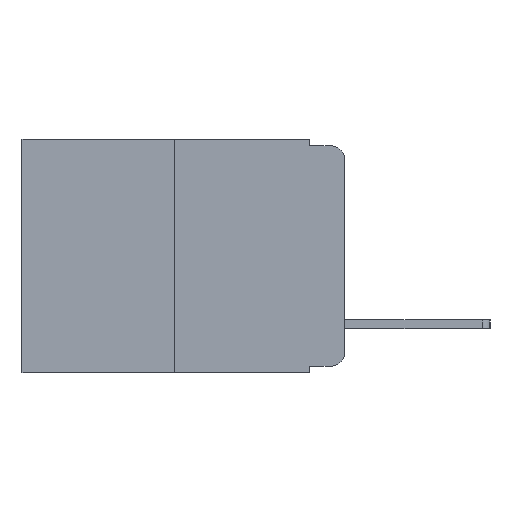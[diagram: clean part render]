
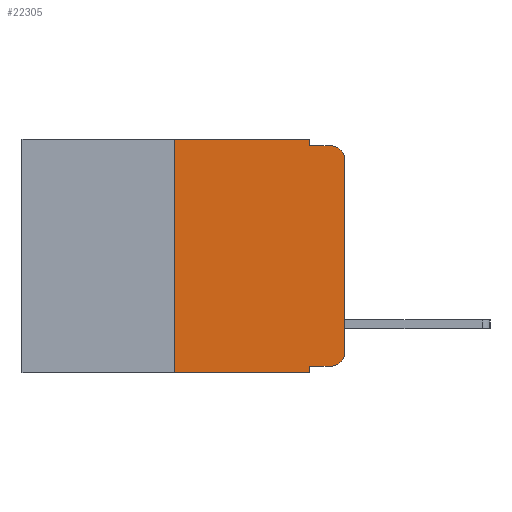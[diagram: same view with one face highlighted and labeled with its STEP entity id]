
A CAD part, left-side view. The second image highlights one B-rep face of the part: STEP entity #22305.
In plain terms, the highlighted planar face has unit normal (-1, 0, 0).
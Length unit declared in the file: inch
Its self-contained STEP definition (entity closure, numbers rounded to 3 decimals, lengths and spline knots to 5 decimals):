
#561 = DIRECTION ( 'NONE',  ( 0., 0., -1. ) ) ;
#583 = DIRECTION ( 'NONE',  ( 0., 0., -1. ) ) ;
#586 = ORIENTED_EDGE ( 'NONE', *, *, #11190, .T. ) ;
#628 = FACE_OUTER_BOUND ( 'NONE', #15506, .T. ) ;
#839 = VECTOR ( 'NONE', #18678, 39.37008 ) ;
#875 = VECTOR ( 'NONE', #18626, 39.37008 ) ;
#943 = VERTEX_POINT ( 'NONE', #12733 ) ;
#1060 = EDGE_CURVE ( 'NONE', #22845, #11990, #15391, .T. ) ;
#1147 = VERTEX_POINT ( 'NONE', #21164 ) ;
#1236 = CARTESIAN_POINT ( 'NONE',  ( 0., 0.473, 0. ) ) ;
#1577 = VECTOR ( 'NONE', #11645, 39.37008 ) ;
#2353 = VERTEX_POINT ( 'NONE', #16899 ) ;
#3320 = ORIENTED_EDGE ( 'NONE', *, *, #8495, .T. ) ;
#3538 = DIRECTION ( 'NONE',  ( 0., 0., 1. ) ) ;
#3705 = ORIENTED_EDGE ( 'NONE', *, *, #23153, .F. ) ;
#3804 = VERTEX_POINT ( 'NONE', #5965 ) ;
#3935 = CARTESIAN_POINT ( 'NONE',  ( 0., 0.25, 0. ) ) ;
#3940 = DIRECTION ( 'NONE',  ( 0., 0., -1. ) ) ;
#4146 = CARTESIAN_POINT ( 'NONE',  ( 0., 0.051, 0. ) ) ;
#4172 = ORIENTED_EDGE ( 'NONE', *, *, #20846, .T. ) ;
#4458 = CARTESIAN_POINT ( 'NONE',  ( 0., 0.051, -0.333 ) ) ;
#4503 = VERTEX_POINT ( 'NONE', #22174 ) ;
#4615 = ORIENTED_EDGE ( 'NONE', *, *, #7274, .F. ) ;
#4837 = EDGE_CURVE ( 'NONE', #2353, #1147, #15476, .T. ) ;
#5032 = ORIENTED_EDGE ( 'NONE', *, *, #19635, .T. ) ;
#5465 = CARTESIAN_POINT ( 'NONE',  ( 0., 0.25, 0. ) ) ;
#5498 = VERTEX_POINT ( 'NONE', #23075 ) ;
#5540 = LINE ( 'NONE', #11544, #10066 ) ;
#5965 = CARTESIAN_POINT ( 'NONE',  ( 0., 0.051, -0.333 ) ) ;
#6021 = CIRCLE ( 'NONE', #8492, 0.02 ) ;
#6303 = DIRECTION ( 'NONE',  ( 0., -1., 0. ) ) ;
#6677 = CARTESIAN_POINT ( 'NONE',  ( 0., 0.02, -0.313 ) ) ;
#7274 = EDGE_CURVE ( 'NONE', #1147, #11995, #19494, .T. ) ;
#7289 = CARTESIAN_POINT ( 'NONE',  ( 0., 0.02, -0.01 ) ) ;
#7557 = CARTESIAN_POINT ( 'NONE',  ( 0., 0.473, 0. ) ) ;
#7959 = VECTOR ( 'NONE', #3538, 39.37008 ) ;
#7970 = CARTESIAN_POINT ( 'NONE',  ( 0., 0.051, -0.01 ) ) ;
#8492 = AXIS2_PLACEMENT_3D ( 'NONE', #6677, #19140, #8506 ) ;
#8495 = EDGE_CURVE ( 'NONE', #943, #11995, #12582, .T. ) ;
#8506 = DIRECTION ( 'NONE',  ( 0., 0., -1. ) ) ;
#9027 = LINE ( 'NONE', #1236, #23147 ) ;
#9638 = VERTEX_POINT ( 'NONE', #10764 ) ;
#10066 = VECTOR ( 'NONE', #583, 39.37008 ) ;
#10335 = ORIENTED_EDGE ( 'NONE', *, *, #1060, .F. ) ;
#10497 = ORIENTED_EDGE ( 'NONE', *, *, #10884, .T. ) ;
#10678 = VECTOR ( 'NONE', #15025, 39.37008 ) ;
#10764 = CARTESIAN_POINT ( 'NONE',  ( 0., 0.02, -0.333 ) ) ;
#10884 = EDGE_CURVE ( 'NONE', #5498, #943, #22094, .T. ) ;
#11190 = EDGE_CURVE ( 'NONE', #22845, #4503, #11302, .T. ) ;
#11302 = LINE ( 'NONE', #13493, #1577 ) ;
#11525 = DIRECTION ( 'NONE',  ( -1., 0., 0. ) ) ;
#11544 = CARTESIAN_POINT ( 'NONE',  ( 0., 0.051, 0. ) ) ;
#11645 = DIRECTION ( 'NONE',  ( 0., -1., 0. ) ) ;
#11908 = AXIS2_PLACEMENT_3D ( 'NONE', #22088, #11525, #561 ) ;
#11990 = VERTEX_POINT ( 'NONE', #5465 ) ;
#11995 = VERTEX_POINT ( 'NONE', #7289 ) ;
#12582 = CIRCLE ( 'NONE', #11908, 0.02 ) ;
#12733 = CARTESIAN_POINT ( 'NONE',  ( 0., 0., -0.03 ) ) ;
#13493 = CARTESIAN_POINT ( 'NONE',  ( 0., 0.473, -0.343 ) ) ;
#14424 = CARTESIAN_POINT ( 'NONE',  ( 0., 0., 0. ) ) ;
#14805 = DIRECTION ( 'NONE',  ( 1., 0., 0. ) ) ;
#15025 = DIRECTION ( 'NONE',  ( 0., 0., -1. ) ) ;
#15391 = LINE ( 'NONE', #3935, #839 ) ;
#15476 = LINE ( 'NONE', #4146, #10678 ) ;
#15506 = EDGE_LOOP ( 'NONE', ( #10497, #3320, #4615, #18058, #18619, #10335, #586, #3705, #4172, #5032 ) ) ;
#16312 = CARTESIAN_POINT ( 'NONE',  ( 0., 0.25, -0.343 ) ) ;
#16899 = CARTESIAN_POINT ( 'NONE',  ( 0., 0.051, 0. ) ) ;
#17158 = LINE ( 'NONE', #4458, #21236 ) ;
#18058 = ORIENTED_EDGE ( 'NONE', *, *, #4837, .F. ) ;
#18619 = ORIENTED_EDGE ( 'NONE', *, *, #20994, .F. ) ;
#18626 = DIRECTION ( 'NONE',  ( 0., -1., 0. ) ) ;
#18678 = DIRECTION ( 'NONE',  ( 0., 0., 1. ) ) ;
#19140 = DIRECTION ( 'NONE',  ( -1., 0., 0. ) ) ;
#19217 = DIRECTION ( 'NONE',  ( 0., -1., 0. ) ) ;
#19494 = LINE ( 'NONE', #7970, #875 ) ;
#19635 = EDGE_CURVE ( 'NONE', #9638, #5498, #6021, .T. ) ;
#19994 = PLANE ( 'NONE',  #21449 ) ;
#20846 = EDGE_CURVE ( 'NONE', #3804, #9638, #17158, .T. ) ;
#20994 = EDGE_CURVE ( 'NONE', #11990, #2353, #9027, .T. ) ;
#21164 = CARTESIAN_POINT ( 'NONE',  ( 0., 0.051, -0.01 ) ) ;
#21236 = VECTOR ( 'NONE', #6303, 39.37008 ) ;
#21449 = AXIS2_PLACEMENT_3D ( 'NONE', #7557, #14805, #3940 ) ;
#22088 = CARTESIAN_POINT ( 'NONE',  ( 0., 0.02, -0.03 ) ) ;
#22094 = LINE ( 'NONE', #14424, #7959 ) ;
#22174 = CARTESIAN_POINT ( 'NONE',  ( 0., 0.051, -0.343 ) ) ;
#22305 = ADVANCED_FACE ( 'NONE', ( #628 ), #19994, .F. ) ;
#22845 = VERTEX_POINT ( 'NONE', #16312 ) ;
#23075 = CARTESIAN_POINT ( 'NONE',  ( 0., 0., -0.313 ) ) ;
#23147 = VECTOR ( 'NONE', #19217, 39.37008 ) ;
#23153 = EDGE_CURVE ( 'NONE', #3804, #4503, #5540, .T. ) ;
